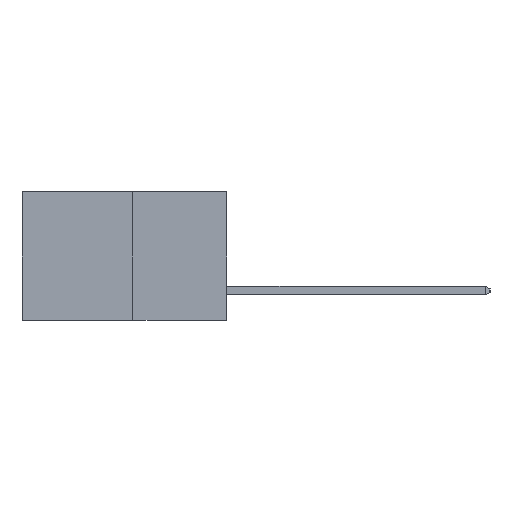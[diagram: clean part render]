
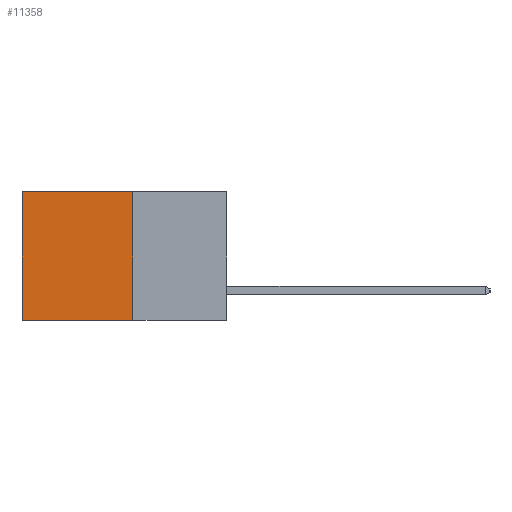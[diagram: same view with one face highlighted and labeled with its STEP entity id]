
A CAD part, left-side view. The second image highlights one B-rep face of the part: STEP entity #11358.
In plain terms, the highlighted planar face has unit normal (-1, 0, 0).
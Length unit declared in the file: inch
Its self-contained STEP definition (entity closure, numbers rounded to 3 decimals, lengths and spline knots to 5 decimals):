
#567 = DIRECTION ( 'NONE',  ( 0., 1., 0. ) ) ;
#1694 = VECTOR ( 'NONE', #3440, 39.37008 ) ;
#2395 = DIRECTION ( 'NONE',  ( 0., 0., -1. ) ) ;
#2722 = LINE ( 'NONE', #8786, #15489 ) ;
#3440 = DIRECTION ( 'NONE',  ( 0., 1., 0. ) ) ;
#3968 = PLANE ( 'NONE',  #17383 ) ;
#4967 = EDGE_CURVE ( 'NONE', #6073, #14720, #15136, .T. ) ;
#6073 = VERTEX_POINT ( 'NONE', #13533 ) ;
#7336 = CARTESIAN_POINT ( 'NONE',  ( 0.277, 0.27, -0.37 ) ) ;
#8786 = CARTESIAN_POINT ( 'NONE',  ( 0.277, 0.27, -0.37 ) ) ;
#8992 = DIRECTION ( 'NONE',  ( 0., 0., -1. ) ) ;
#9048 = VERTEX_POINT ( 'NONE', #17937 ) ;
#9566 = DIRECTION ( 'NONE',  ( 0., 0., -1. ) ) ;
#9596 = CARTESIAN_POINT ( 'NONE',  ( 0.277, 0.59, -0.37 ) ) ;
#9609 = VECTOR ( 'NONE', #2395, 39.37008 ) ;
#9636 = EDGE_LOOP ( 'NONE', ( #20574, #10691, #12717, #10738 ) ) ;
#9661 = CARTESIAN_POINT ( 'NONE',  ( 0.277, 0.59, -0.37 ) ) ;
#9875 = EDGE_CURVE ( 'NONE', #19397, #6073, #14472, .T. ) ;
#10151 = VECTOR ( 'NONE', #9566, 39.37008 ) ;
#10201 = FACE_OUTER_BOUND ( 'NONE', #9636, .T. ) ;
#10691 = ORIENTED_EDGE ( 'NONE', *, *, #18675, .F. ) ;
#10738 = ORIENTED_EDGE ( 'NONE', *, *, #9875, .T. ) ;
#11358 = ADVANCED_FACE ( 'NONE', ( #10201 ), #3968, .F. ) ;
#12308 = CARTESIAN_POINT ( 'NONE',  ( 0.277, 0.27, -0.37 ) ) ;
#12717 = ORIENTED_EDGE ( 'NONE', *, *, #13426, .F. ) ;
#13426 = EDGE_CURVE ( 'NONE', #19397, #9048, #14071, .T. ) ;
#13533 = CARTESIAN_POINT ( 'NONE',  ( 0.277, 0.59, 0. ) ) ;
#14071 = LINE ( 'NONE', #12308, #9609 ) ;
#14472 = LINE ( 'NONE', #20074, #1694 ) ;
#14720 = VERTEX_POINT ( 'NONE', #9596 ) ;
#15136 = LINE ( 'NONE', #9661, #10151 ) ;
#15489 = VECTOR ( 'NONE', #567, 39.37008 ) ;
#17383 = AXIS2_PLACEMENT_3D ( 'NONE', #7336, #19029, #8992 ) ;
#17937 = CARTESIAN_POINT ( 'NONE',  ( 0.277, 0.27, -0.37 ) ) ;
#18675 = EDGE_CURVE ( 'NONE', #9048, #14720, #2722, .T. ) ;
#19029 = DIRECTION ( 'NONE',  ( 1., 0., 0. ) ) ;
#19397 = VERTEX_POINT ( 'NONE', #20865 ) ;
#20074 = CARTESIAN_POINT ( 'NONE',  ( 0.277, 0.27, 0. ) ) ;
#20574 = ORIENTED_EDGE ( 'NONE', *, *, #4967, .T. ) ;
#20865 = CARTESIAN_POINT ( 'NONE',  ( 0.277, 0.27, 0. ) ) ;
